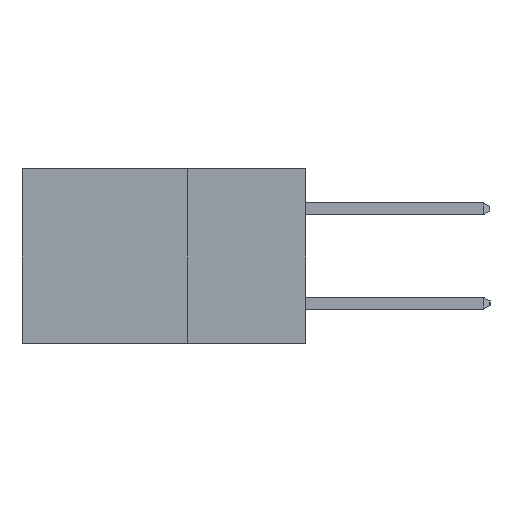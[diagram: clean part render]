
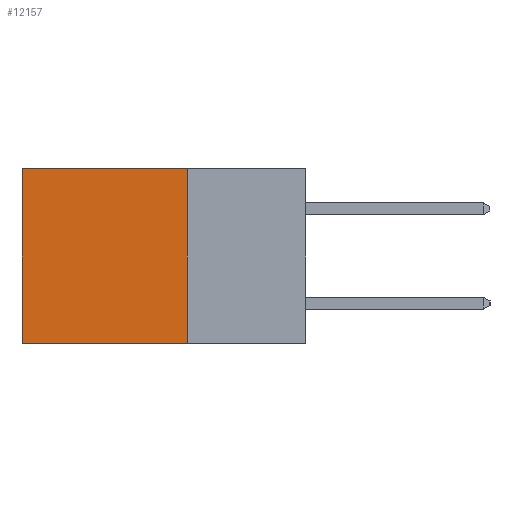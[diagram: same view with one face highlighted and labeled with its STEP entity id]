
A CAD part, left-side view. The second image highlights one B-rep face of the part: STEP entity #12157.
In plain terms, the highlighted planar face has unit normal (-1, 0, 0).
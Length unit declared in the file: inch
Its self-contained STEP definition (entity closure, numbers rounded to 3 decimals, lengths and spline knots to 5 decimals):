
#147 = DIRECTION ( 'NONE',  ( 0., 1., 0. ) ) ;
#1099 = VERTEX_POINT ( 'NONE', #10961 ) ;
#1373 = VECTOR ( 'NONE', #8957, 39.37008 ) ;
#1463 = CARTESIAN_POINT ( 'NONE',  ( 0.2615, 0.25, 0. ) ) ;
#1535 = LINE ( 'NONE', #14231, #8552 ) ;
#1924 = VERTEX_POINT ( 'NONE', #13674 ) ;
#2932 = CARTESIAN_POINT ( 'NONE',  ( 0.2615, 0.6, 0. ) ) ;
#3919 = FACE_OUTER_BOUND ( 'NONE', #8822, .T. ) ;
#5179 = ORIENTED_EDGE ( 'NONE', *, *, #6509, .T. ) ;
#6094 = DIRECTION ( 'NONE',  ( 0., 0., -1. ) ) ;
#6509 = EDGE_CURVE ( 'NONE', #1099, #13878, #6955, .T. ) ;
#6955 = LINE ( 'NONE', #1463, #10214 ) ;
#8446 = DIRECTION ( 'NONE',  ( 0., 1., 0. ) ) ;
#8552 = VECTOR ( 'NONE', #15585, 39.37008 ) ;
#8564 = CARTESIAN_POINT ( 'NONE',  ( 0.2615, 0.25, -0.37 ) ) ;
#8567 = AXIS2_PLACEMENT_3D ( 'NONE', #16999, #14407, #6094 ) ;
#8822 = EDGE_LOOP ( 'NONE', ( #15297, #11516, #11436, #5179 ) ) ;
#8957 = DIRECTION ( 'NONE',  ( 0., 0., -1. ) ) ;
#9563 = EDGE_CURVE ( 'NONE', #1099, #13759, #12534, .T. ) ;
#9674 = CARTESIAN_POINT ( 'NONE',  ( 0.2615, 0.25, -0.37 ) ) ;
#10214 = VECTOR ( 'NONE', #8446, 39.37008 ) ;
#10217 = PLANE ( 'NONE',  #8567 ) ;
#10350 = CARTESIAN_POINT ( 'NONE',  ( 0.2615, 0.25, -0.37 ) ) ;
#10961 = CARTESIAN_POINT ( 'NONE',  ( 0.2615, 0.25, 0. ) ) ;
#11436 = ORIENTED_EDGE ( 'NONE', *, *, #9563, .F. ) ;
#11516 = ORIENTED_EDGE ( 'NONE', *, *, #17936, .F. ) ;
#11535 = LINE ( 'NONE', #8564, #15611 ) ;
#12068 = EDGE_CURVE ( 'NONE', #13878, #1924, #1535, .T. ) ;
#12157 = ADVANCED_FACE ( 'NONE', ( #3919 ), #10217, .F. ) ;
#12534 = LINE ( 'NONE', #10350, #1373 ) ;
#13674 = CARTESIAN_POINT ( 'NONE',  ( 0.2615, 0.6, -0.37 ) ) ;
#13759 = VERTEX_POINT ( 'NONE', #9674 ) ;
#13878 = VERTEX_POINT ( 'NONE', #2932 ) ;
#14231 = CARTESIAN_POINT ( 'NONE',  ( 0.2615, 0.6, -0.37 ) ) ;
#14407 = DIRECTION ( 'NONE',  ( 1., 0., 0. ) ) ;
#15297 = ORIENTED_EDGE ( 'NONE', *, *, #12068, .T. ) ;
#15585 = DIRECTION ( 'NONE',  ( 0., 0., -1. ) ) ;
#15611 = VECTOR ( 'NONE', #147, 39.37008 ) ;
#16999 = CARTESIAN_POINT ( 'NONE',  ( 0.2615, 0.25, -0.37 ) ) ;
#17936 = EDGE_CURVE ( 'NONE', #13759, #1924, #11535, .T. ) ;
